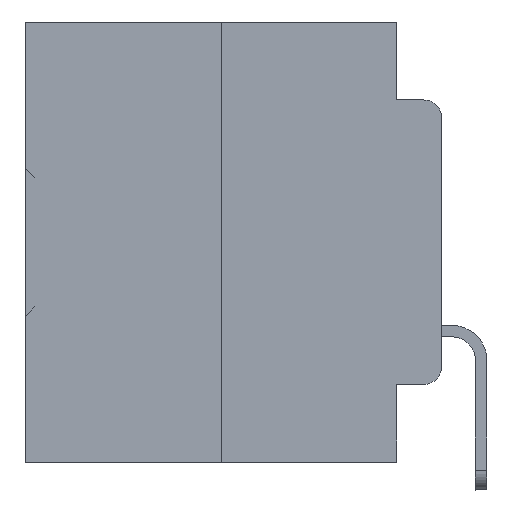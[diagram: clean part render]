
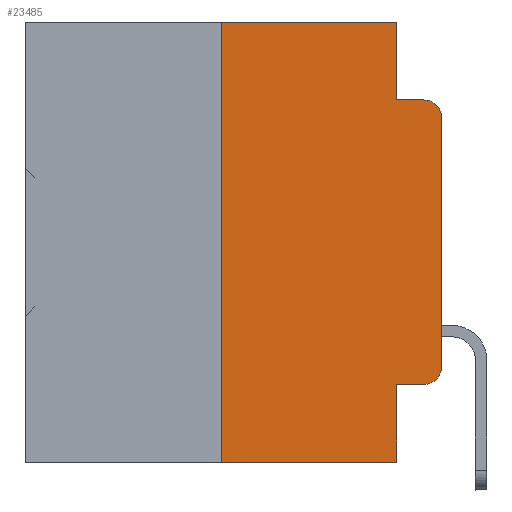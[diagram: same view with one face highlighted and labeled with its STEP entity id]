
A CAD part, left-side view. The second image highlights one B-rep face of the part: STEP entity #23485.
In plain terms, the highlighted planar face has unit normal (-1, 0, 0).
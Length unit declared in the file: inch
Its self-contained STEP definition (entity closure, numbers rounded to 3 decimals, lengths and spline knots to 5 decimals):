
#123 = CARTESIAN_POINT ( 'NONE',  ( 0., 0.051, 0. ) ) ;
#323 = DIRECTION ( 'NONE',  ( 0., 0., 1. ) ) ;
#472 = LINE ( 'NONE', #29145, #17609 ) ;
#522 = EDGE_CURVE ( 'NONE', #15427, #20919, #28807, .T. ) ;
#608 = VERTEX_POINT ( 'NONE', #26109 ) ;
#1082 = CARTESIAN_POINT ( 'NONE',  ( 0., 0.02, -0.0885 ) ) ;
#1682 = DIRECTION ( 'NONE',  ( 0., 0., -1. ) ) ;
#2262 = DIRECTION ( 'NONE',  ( 0., 0., -1. ) ) ;
#2338 = EDGE_CURVE ( 'NONE', #608, #20919, #472, .T. ) ;
#2417 = VECTOR ( 'NONE', #2262, 39.37008 ) ;
#2817 = VERTEX_POINT ( 'NONE', #14460 ) ;
#3186 = ORIENTED_EDGE ( 'NONE', *, *, #522, .F. ) ;
#3606 = CARTESIAN_POINT ( 'NONE',  ( 0., 0.051, 0. ) ) ;
#4251 = VECTOR ( 'NONE', #14112, 39.37008 ) ;
#5729 = AXIS2_PLACEMENT_3D ( 'NONE', #33369, #21631, #36071 ) ;
#6688 = DIRECTION ( 'NONE',  ( -1., 0., 0. ) ) ;
#6736 = ORIENTED_EDGE ( 'NONE', *, *, #34615, .F. ) ;
#6829 = CARTESIAN_POINT ( 'NONE',  ( 0., 0.051, -0.0885 ) ) ;
#7267 = ORIENTED_EDGE ( 'NONE', *, *, #18927, .F. ) ;
#7462 = DIRECTION ( 'NONE',  ( -1., 0., 0. ) ) ;
#8063 = CARTESIAN_POINT ( 'NONE',  ( 0., 0.051, -0.4115 ) ) ;
#8350 = ORIENTED_EDGE ( 'NONE', *, *, #21665, .T. ) ;
#8427 = DIRECTION ( 'NONE',  ( 0., -1., 0. ) ) ;
#9390 = VECTOR ( 'NONE', #34621, 39.37008 ) ;
#9525 = VERTEX_POINT ( 'NONE', #25794 ) ;
#11303 = LINE ( 'NONE', #23048, #15542 ) ;
#11718 = ORIENTED_EDGE ( 'NONE', *, *, #18945, .T. ) ;
#11729 = LINE ( 'NONE', #23467, #9390 ) ;
#12250 = CARTESIAN_POINT ( 'NONE',  ( 0., 0., 0. ) ) ;
#14112 = DIRECTION ( 'NONE',  ( 0., -1., 0. ) ) ;
#14460 = CARTESIAN_POINT ( 'NONE',  ( 0., 0., -0.3915 ) ) ;
#15284 = CIRCLE ( 'NONE', #26327, 0.02 ) ;
#15329 = CARTESIAN_POINT ( 'NONE',  ( 0., 0.02, -0.3915 ) ) ;
#15427 = VERTEX_POINT ( 'NONE', #8063 ) ;
#15542 = VECTOR ( 'NONE', #8427, 39.37008 ) ;
#16425 = ORIENTED_EDGE ( 'NONE', *, *, #29333, .T. ) ;
#16995 = LINE ( 'NONE', #28749, #4251 ) ;
#17609 = VECTOR ( 'NONE', #23186, 39.37008 ) ;
#17788 = EDGE_CURVE ( 'NONE', #2817, #34855, #33020, .T. ) ;
#18252 = VERTEX_POINT ( 'NONE', #6829 ) ;
#18927 = EDGE_CURVE ( 'NONE', #30790, #18252, #29193, .T. ) ;
#18945 = EDGE_CURVE ( 'NONE', #20396, #2817, #15284, .T. ) ;
#19998 = LINE ( 'NONE', #25609, #25927 ) ;
#20396 = VERTEX_POINT ( 'NONE', #21301 ) ;
#20404 = ORIENTED_EDGE ( 'NONE', *, *, #17788, .T. ) ;
#20788 = VECTOR ( 'NONE', #23991, 39.37008 ) ;
#20857 = ORIENTED_EDGE ( 'NONE', *, *, #34081, .F. ) ;
#20919 = VERTEX_POINT ( 'NONE', #28739 ) ;
#20969 = ORIENTED_EDGE ( 'NONE', *, *, #2338, .T. ) ;
#21098 = DIRECTION ( 'NONE',  ( 0., 0., -1. ) ) ;
#21301 = CARTESIAN_POINT ( 'NONE',  ( 0., 0.02, -0.4115 ) ) ;
#21631 = DIRECTION ( 'NONE',  ( 1., 0., 0. ) ) ;
#21665 = EDGE_CURVE ( 'NONE', #34855, #30842, #34496, .T. ) ;
#22078 = CARTESIAN_POINT ( 'NONE',  ( 0., 0.02, -0.1085 ) ) ;
#22462 = FACE_OUTER_BOUND ( 'NONE', #30230, .T. ) ;
#23048 = CARTESIAN_POINT ( 'NONE',  ( 0., 0.473, 0. ) ) ;
#23186 = DIRECTION ( 'NONE',  ( 0., -1., 0. ) ) ;
#23467 = CARTESIAN_POINT ( 'NONE',  ( 0., 0.051, -0.0885 ) ) ;
#23485 = ADVANCED_FACE ( 'NONE', ( #22462 ), #30505, .F. ) ;
#23991 = DIRECTION ( 'NONE',  ( 0., 0., -1. ) ) ;
#25609 = CARTESIAN_POINT ( 'NONE',  ( 0., 0.25, 0. ) ) ;
#25794 = CARTESIAN_POINT ( 'NONE',  ( 0., 0.25, 0. ) ) ;
#25927 = VECTOR ( 'NONE', #31189, 39.37008 ) ;
#26109 = CARTESIAN_POINT ( 'NONE',  ( 0., 0.25, -0.5 ) ) ;
#26327 = AXIS2_PLACEMENT_3D ( 'NONE', #15329, #6688, #21098 ) ;
#28365 = AXIS2_PLACEMENT_3D ( 'NONE', #22078, #7462, #1682 ) ;
#28622 = CARTESIAN_POINT ( 'NONE',  ( 0., 0.051, 0. ) ) ;
#28739 = CARTESIAN_POINT ( 'NONE',  ( 0., 0.051, -0.5 ) ) ;
#28749 = CARTESIAN_POINT ( 'NONE',  ( 0., 0.051, -0.4115 ) ) ;
#28807 = LINE ( 'NONE', #28622, #2417 ) ;
#29145 = CARTESIAN_POINT ( 'NONE',  ( 0., 0.473, -0.5 ) ) ;
#29193 = LINE ( 'NONE', #3606, #20788 ) ;
#29238 = ORIENTED_EDGE ( 'NONE', *, *, #35299, .F. ) ;
#29333 = EDGE_CURVE ( 'NONE', #15427, #20396, #16995, .T. ) ;
#30230 = EDGE_LOOP ( 'NONE', ( #20404, #8350, #20857, #7267, #6736, #29238, #20969, #3186, #16425, #11718 ) ) ;
#30505 = PLANE ( 'NONE',  #5729 ) ;
#30790 = VERTEX_POINT ( 'NONE', #123 ) ;
#30842 = VERTEX_POINT ( 'NONE', #1082 ) ;
#31189 = DIRECTION ( 'NONE',  ( 0., 0., 1. ) ) ;
#33020 = LINE ( 'NONE', #12250, #33115 ) ;
#33115 = VECTOR ( 'NONE', #323, 39.37008 ) ;
#33369 = CARTESIAN_POINT ( 'NONE',  ( 0., 0.473, 0. ) ) ;
#33408 = CARTESIAN_POINT ( 'NONE',  ( 0., 0., -0.1085 ) ) ;
#34081 = EDGE_CURVE ( 'NONE', #18252, #30842, #11729, .T. ) ;
#34496 = CIRCLE ( 'NONE', #28365, 0.02 ) ;
#34615 = EDGE_CURVE ( 'NONE', #9525, #30790, #11303, .T. ) ;
#34621 = DIRECTION ( 'NONE',  ( 0., -1., 0. ) ) ;
#34855 = VERTEX_POINT ( 'NONE', #33408 ) ;
#35299 = EDGE_CURVE ( 'NONE', #608, #9525, #19998, .T. ) ;
#36071 = DIRECTION ( 'NONE',  ( 0., 0., -1. ) ) ;
